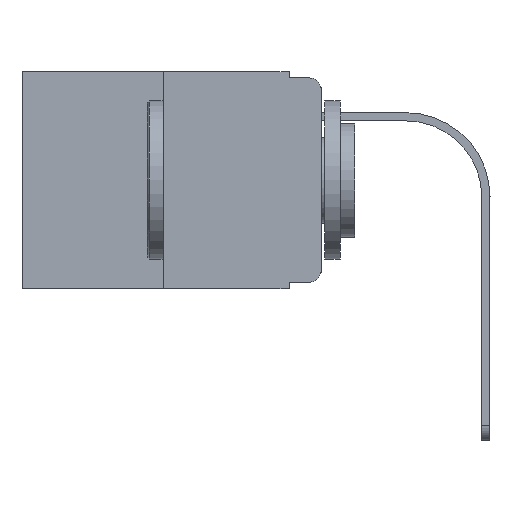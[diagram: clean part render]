
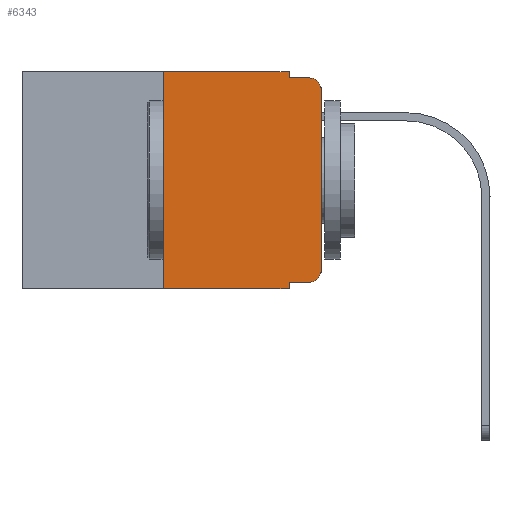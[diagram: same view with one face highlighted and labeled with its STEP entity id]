
A CAD part, left-side view. The second image highlights one B-rep face of the part: STEP entity #6343.
In plain terms, the highlighted planar face has unit normal (-1, 0, 0).
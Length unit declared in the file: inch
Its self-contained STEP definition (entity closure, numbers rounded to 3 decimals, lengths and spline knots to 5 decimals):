
#269 = CARTESIAN_POINT ( 'NONE',  ( 0., 0.051, -0.01 ) ) ;
#361 = ORIENTED_EDGE ( 'NONE', *, *, #517, .F. ) ;
#517 = EDGE_CURVE ( 'NONE', #19702, #19651, #4322, .T. ) ;
#530 = DIRECTION ( 'NONE',  ( 0., 0., -1. ) ) ;
#579 = AXIS2_PLACEMENT_3D ( 'NONE', #15168, #21649, #13720 ) ;
#734 = DIRECTION ( 'NONE',  ( 0., -1., 0. ) ) ;
#910 = ORIENTED_EDGE ( 'NONE', *, *, #9777, .T. ) ;
#948 = CARTESIAN_POINT ( 'NONE',  ( 0., 0.473, 0. ) ) ;
#950 = ORIENTED_EDGE ( 'NONE', *, *, #15464, .T. ) ;
#975 = DIRECTION ( 'NONE',  ( -1., 0., 0. ) ) ;
#1159 = VECTOR ( 'NONE', #21230, 39.37008 ) ;
#1290 = EDGE_LOOP ( 'NONE', ( #910, #14829, #3371, #9455, #7696, #9571, #6327, #361, #950, #3487 ) ) ;
#1858 = CARTESIAN_POINT ( 'NONE',  ( 0., 0.02, -0.313 ) ) ;
#2048 = VERTEX_POINT ( 'NONE', #15458 ) ;
#2384 = EDGE_CURVE ( 'NONE', #12470, #12001, #2478, .T. ) ;
#2458 = CARTESIAN_POINT ( 'NONE',  ( 0., 0.051, 0. ) ) ;
#2478 = CIRCLE ( 'NONE', #16929, 0.02 ) ;
#2491 = LINE ( 'NONE', #948, #3584 ) ;
#2561 = VERTEX_POINT ( 'NONE', #17846 ) ;
#2602 = VECTOR ( 'NONE', #20250, 39.37008 ) ;
#3070 = EDGE_CURVE ( 'NONE', #5882, #11399, #2491, .T. ) ;
#3309 = DIRECTION ( 'NONE',  ( 0., 0., 1. ) ) ;
#3371 = ORIENTED_EDGE ( 'NONE', *, *, #21676, .F. ) ;
#3487 = ORIENTED_EDGE ( 'NONE', *, *, #2384, .T. ) ;
#3584 = VECTOR ( 'NONE', #19573, 39.37008 ) ;
#3925 = CARTESIAN_POINT ( 'NONE',  ( 0., 0.051, 0. ) ) ;
#4016 = EDGE_CURVE ( 'NONE', #2048, #19651, #9798, .T. ) ;
#4276 = VERTEX_POINT ( 'NONE', #10976 ) ;
#4322 = LINE ( 'NONE', #2458, #13183 ) ;
#4821 = CARTESIAN_POINT ( 'NONE',  ( 0., 0.02, -0.03 ) ) ;
#5717 = CARTESIAN_POINT ( 'NONE',  ( 0., 0.051, -0.333 ) ) ;
#5882 = VERTEX_POINT ( 'NONE', #6591 ) ;
#6327 = ORIENTED_EDGE ( 'NONE', *, *, #4016, .T. ) ;
#6343 = ADVANCED_FACE ( 'NONE', ( #16832 ), #8445, .F. ) ;
#6591 = CARTESIAN_POINT ( 'NONE',  ( 0., 0.25, 0. ) ) ;
#7337 = VECTOR ( 'NONE', #20900, 39.37008 ) ;
#7696 = ORIENTED_EDGE ( 'NONE', *, *, #3070, .F. ) ;
#8429 = VECTOR ( 'NONE', #3309, 39.37008 ) ;
#8445 = PLANE ( 'NONE',  #579 ) ;
#9189 = DIRECTION ( 'NONE',  ( 0., 0., -1. ) ) ;
#9455 = ORIENTED_EDGE ( 'NONE', *, *, #18891, .F. ) ;
#9562 = CARTESIAN_POINT ( 'NONE',  ( 0., 0., 0. ) ) ;
#9571 = ORIENTED_EDGE ( 'NONE', *, *, #19418, .F. ) ;
#9777 = EDGE_CURVE ( 'NONE', #12001, #2561, #21345, .T. ) ;
#9798 = LINE ( 'NONE', #11663, #2602 ) ;
#9832 = CARTESIAN_POINT ( 'NONE',  ( 0., 0.25, 0. ) ) ;
#10154 = CARTESIAN_POINT ( 'NONE',  ( 0., 0.051, -0.343 ) ) ;
#10976 = CARTESIAN_POINT ( 'NONE',  ( 0., 0.051, -0.01 ) ) ;
#11073 = CARTESIAN_POINT ( 'NONE',  ( 0., 0.02, -0.333 ) ) ;
#11399 = VERTEX_POINT ( 'NONE', #12517 ) ;
#11663 = CARTESIAN_POINT ( 'NONE',  ( 0., 0.473, -0.343 ) ) ;
#12001 = VERTEX_POINT ( 'NONE', #16760 ) ;
#12291 = VERTEX_POINT ( 'NONE', #13084 ) ;
#12470 = VERTEX_POINT ( 'NONE', #11073 ) ;
#12517 = CARTESIAN_POINT ( 'NONE',  ( 0., 0.051, 0. ) ) ;
#13084 = CARTESIAN_POINT ( 'NONE',  ( 0., 0.02, -0.01 ) ) ;
#13183 = VECTOR ( 'NONE', #9189, 39.37008 ) ;
#13252 = VECTOR ( 'NONE', #734, 39.37008 ) ;
#13577 = CIRCLE ( 'NONE', #19566, 0.02 ) ;
#13720 = DIRECTION ( 'NONE',  ( 0., 0., -1. ) ) ;
#14418 = VECTOR ( 'NONE', #15262, 39.37008 ) ;
#14798 = LINE ( 'NONE', #9832, #8429 ) ;
#14829 = ORIENTED_EDGE ( 'NONE', *, *, #15226, .T. ) ;
#15168 = CARTESIAN_POINT ( 'NONE',  ( 0., 0.473, 0. ) ) ;
#15226 = EDGE_CURVE ( 'NONE', #2561, #12291, #13577, .T. ) ;
#15262 = DIRECTION ( 'NONE',  ( 0., -1., 0. ) ) ;
#15458 = CARTESIAN_POINT ( 'NONE',  ( 0., 0.25, -0.343 ) ) ;
#15464 = EDGE_CURVE ( 'NONE', #19702, #12470, #20565, .T. ) ;
#15534 = DIRECTION ( 'NONE',  ( -1., 0., 0. ) ) ;
#15705 = LINE ( 'NONE', #269, #14418 ) ;
#15956 = CARTESIAN_POINT ( 'NONE',  ( 0., 0.051, -0.333 ) ) ;
#16309 = DIRECTION ( 'NONE',  ( 0., 0., -1. ) ) ;
#16760 = CARTESIAN_POINT ( 'NONE',  ( 0., 0., -0.313 ) ) ;
#16832 = FACE_OUTER_BOUND ( 'NONE', #1290, .T. ) ;
#16929 = AXIS2_PLACEMENT_3D ( 'NONE', #1858, #15534, #530 ) ;
#17298 = LINE ( 'NONE', #3925, #7337 ) ;
#17846 = CARTESIAN_POINT ( 'NONE',  ( 0., 0., -0.03 ) ) ;
#18891 = EDGE_CURVE ( 'NONE', #11399, #4276, #17298, .T. ) ;
#19418 = EDGE_CURVE ( 'NONE', #2048, #5882, #14798, .T. ) ;
#19566 = AXIS2_PLACEMENT_3D ( 'NONE', #4821, #975, #16309 ) ;
#19573 = DIRECTION ( 'NONE',  ( 0., -1., 0. ) ) ;
#19651 = VERTEX_POINT ( 'NONE', #10154 ) ;
#19702 = VERTEX_POINT ( 'NONE', #5717 ) ;
#20250 = DIRECTION ( 'NONE',  ( 0., -1., 0. ) ) ;
#20565 = LINE ( 'NONE', #15956, #13252 ) ;
#20900 = DIRECTION ( 'NONE',  ( 0., 0., -1. ) ) ;
#21230 = DIRECTION ( 'NONE',  ( 0., 0., 1. ) ) ;
#21345 = LINE ( 'NONE', #9562, #1159 ) ;
#21649 = DIRECTION ( 'NONE',  ( 1., 0., 0. ) ) ;
#21676 = EDGE_CURVE ( 'NONE', #4276, #12291, #15705, .T. ) ;
